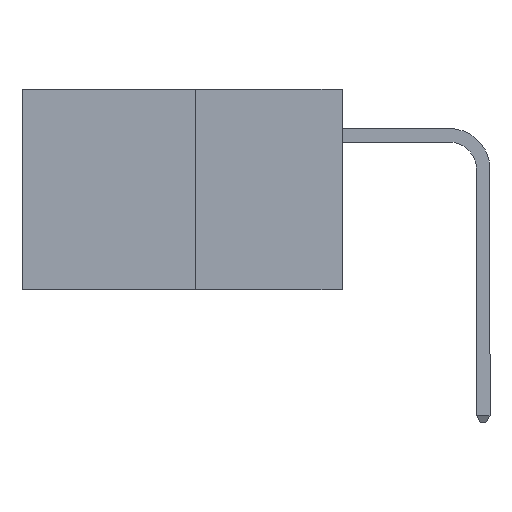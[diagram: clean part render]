
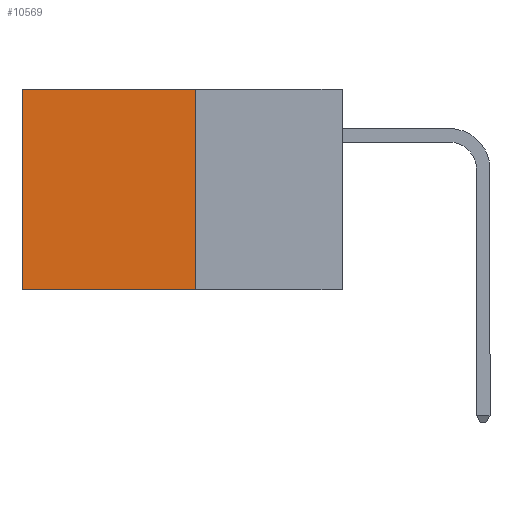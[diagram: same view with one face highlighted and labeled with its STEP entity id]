
A CAD part, left-side view. The second image highlights one B-rep face of the part: STEP entity #10569.
In plain terms, the highlighted planar face has unit normal (-1, 0, 0).
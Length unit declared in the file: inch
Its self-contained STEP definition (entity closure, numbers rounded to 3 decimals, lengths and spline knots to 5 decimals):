
#1030 = VERTEX_POINT ( 'NONE', #16444 ) ;
#1396 = PLANE ( 'NONE',  #11037 ) ;
#1542 = VECTOR ( 'NONE', #5511, 39.37008 ) ;
#2432 = ORIENTED_EDGE ( 'NONE', *, *, #9152, .T. ) ;
#2628 = CARTESIAN_POINT ( 'NONE',  ( 0.277, 0.59, -0.37 ) ) ;
#2859 = CARTESIAN_POINT ( 'NONE',  ( 0.277, 0.27, 0. ) ) ;
#3270 = CARTESIAN_POINT ( 'NONE',  ( 0.277, 0.59, 0. ) ) ;
#4142 = DIRECTION ( 'NONE',  ( 0., 0., -1. ) ) ;
#4613 = CARTESIAN_POINT ( 'NONE',  ( 0.277, 0.27, -0.37 ) ) ;
#4769 = CARTESIAN_POINT ( 'NONE',  ( 0.277, 0.59, -0.37 ) ) ;
#4824 = VECTOR ( 'NONE', #7278, 39.37008 ) ;
#4944 = FACE_OUTER_BOUND ( 'NONE', #11718, .T. ) ;
#5230 = VECTOR ( 'NONE', #4142, 39.37008 ) ;
#5356 = CARTESIAN_POINT ( 'NONE',  ( 0.277, 0.27, -0.37 ) ) ;
#5511 = DIRECTION ( 'NONE',  ( 0., 1., 0. ) ) ;
#5686 = VERTEX_POINT ( 'NONE', #2628 ) ;
#6698 = DIRECTION ( 'NONE',  ( 0., 0., -1. ) ) ;
#7278 = DIRECTION ( 'NONE',  ( 0., 1., 0. ) ) ;
#7451 = CARTESIAN_POINT ( 'NONE',  ( 0.277, 0.27, -0.37 ) ) ;
#7620 = ORIENTED_EDGE ( 'NONE', *, *, #14050, .F. ) ;
#8107 = CARTESIAN_POINT ( 'NONE',  ( 0.277, 0.27, -0.37 ) ) ;
#8146 = VECTOR ( 'NONE', #12739, 39.37008 ) ;
#8774 = LINE ( 'NONE', #8107, #5230 ) ;
#8790 = LINE ( 'NONE', #4613, #4824 ) ;
#9152 = EDGE_CURVE ( 'NONE', #10825, #5686, #11273, .T. ) ;
#10569 = ADVANCED_FACE ( 'NONE', ( #4944 ), #1396, .F. ) ;
#10825 = VERTEX_POINT ( 'NONE', #3270 ) ;
#11037 = AXIS2_PLACEMENT_3D ( 'NONE', #5356, #14664, #6698 ) ;
#11273 = LINE ( 'NONE', #4769, #8146 ) ;
#11718 = EDGE_LOOP ( 'NONE', ( #2432, #7620, #16542, #13009 ) ) ;
#12257 = VERTEX_POINT ( 'NONE', #7451 ) ;
#12739 = DIRECTION ( 'NONE',  ( 0., 0., -1. ) ) ;
#13009 = ORIENTED_EDGE ( 'NONE', *, *, #13161, .T. ) ;
#13161 = EDGE_CURVE ( 'NONE', #1030, #10825, #16074, .T. ) ;
#14050 = EDGE_CURVE ( 'NONE', #12257, #5686, #8790, .T. ) ;
#14469 = EDGE_CURVE ( 'NONE', #1030, #12257, #8774, .T. ) ;
#14664 = DIRECTION ( 'NONE',  ( 1., 0., 0. ) ) ;
#16074 = LINE ( 'NONE', #2859, #1542 ) ;
#16444 = CARTESIAN_POINT ( 'NONE',  ( 0.277, 0.27, 0. ) ) ;
#16542 = ORIENTED_EDGE ( 'NONE', *, *, #14469, .F. ) ;
